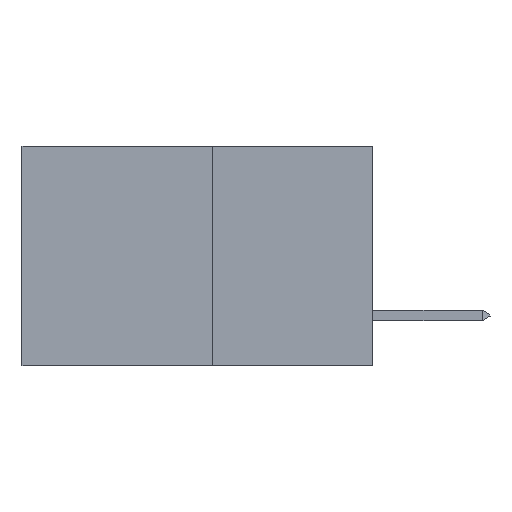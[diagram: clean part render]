
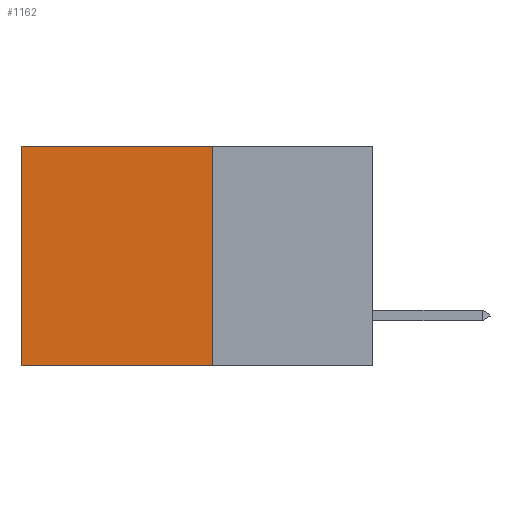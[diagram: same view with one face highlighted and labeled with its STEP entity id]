
A CAD part, left-side view. The second image highlights one B-rep face of the part: STEP entity #1162.
In plain terms, the highlighted planar face has unit normal (-1, 0, 0).
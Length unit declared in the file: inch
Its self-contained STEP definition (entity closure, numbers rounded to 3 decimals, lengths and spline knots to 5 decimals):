
#245 = CARTESIAN_POINT ( 'NONE',  ( 0.277, 0.27, -0.37 ) ) ;
#363 = DIRECTION ( 'NONE',  ( 0., 0., -1. ) ) ;
#404 = DIRECTION ( 'NONE',  ( 1., 0., 0. ) ) ;
#426 = DIRECTION ( 'NONE',  ( 0., 1., 0. ) ) ;
#453 = CARTESIAN_POINT ( 'NONE',  ( 0.277, 0.59, 0. ) ) ;
#515 = CARTESIAN_POINT ( 'NONE',  ( 0.277, 0.27, -0.37 ) ) ;
#692 = CARTESIAN_POINT ( 'NONE',  ( 0.277, 0.27, -0.37 ) ) ;
#711 = EDGE_CURVE ( 'NONE', #7529, #3078, #1544, .T. ) ;
#717 = PLANE ( 'NONE',  #10496 ) ;
#833 = DIRECTION ( 'NONE',  ( 0., 0., -1. ) ) ;
#1162 = ADVANCED_FACE ( 'NONE', ( #9110 ), #717, .F. ) ;
#1172 = ORIENTED_EDGE ( 'NONE', *, *, #1950, .T. ) ;
#1228 = ORIENTED_EDGE ( 'NONE', *, *, #711, .F. ) ;
#1278 = DIRECTION ( 'NONE',  ( 0., 0., -1. ) ) ;
#1401 = CARTESIAN_POINT ( 'NONE',  ( 0.277, 0.59, -0.37 ) ) ;
#1544 = LINE ( 'NONE', #515, #10445 ) ;
#1950 = EDGE_CURVE ( 'NONE', #13709, #3078, #4698, .T. ) ;
#2056 = VECTOR ( 'NONE', #1278, 39.37008 ) ;
#3078 = VERTEX_POINT ( 'NONE', #1401 ) ;
#3131 = VECTOR ( 'NONE', #12525, 39.37008 ) ;
#4553 = CARTESIAN_POINT ( 'NONE',  ( 0.277, 0.27, 0. ) ) ;
#4698 = LINE ( 'NONE', #9431, #10089 ) ;
#5044 = EDGE_CURVE ( 'NONE', #12882, #7529, #10635, .T. ) ;
#5544 = ORIENTED_EDGE ( 'NONE', *, *, #5044, .F. ) ;
#7529 = VERTEX_POINT ( 'NONE', #10590 ) ;
#9110 = FACE_OUTER_BOUND ( 'NONE', #11639, .T. ) ;
#9366 = EDGE_CURVE ( 'NONE', #12882, #13709, #11986, .T. ) ;
#9431 = CARTESIAN_POINT ( 'NONE',  ( 0.277, 0.59, -0.37 ) ) ;
#10089 = VECTOR ( 'NONE', #833, 39.37008 ) ;
#10445 = VECTOR ( 'NONE', #426, 39.37008 ) ;
#10496 = AXIS2_PLACEMENT_3D ( 'NONE', #692, #404, #363 ) ;
#10590 = CARTESIAN_POINT ( 'NONE',  ( 0.277, 0.27, -0.37 ) ) ;
#10635 = LINE ( 'NONE', #245, #2056 ) ;
#11475 = CARTESIAN_POINT ( 'NONE',  ( 0.277, 0.27, 0. ) ) ;
#11639 = EDGE_LOOP ( 'NONE', ( #1172, #1228, #5544, #13652 ) ) ;
#11986 = LINE ( 'NONE', #11475, #3131 ) ;
#12525 = DIRECTION ( 'NONE',  ( 0., 1., 0. ) ) ;
#12882 = VERTEX_POINT ( 'NONE', #4553 ) ;
#13652 = ORIENTED_EDGE ( 'NONE', *, *, #9366, .T. ) ;
#13709 = VERTEX_POINT ( 'NONE', #453 ) ;
